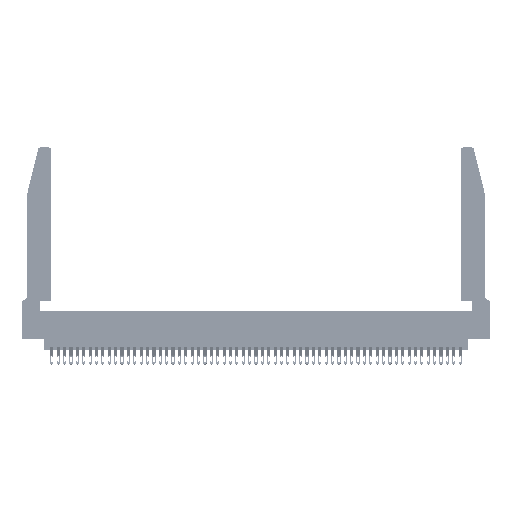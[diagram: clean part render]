
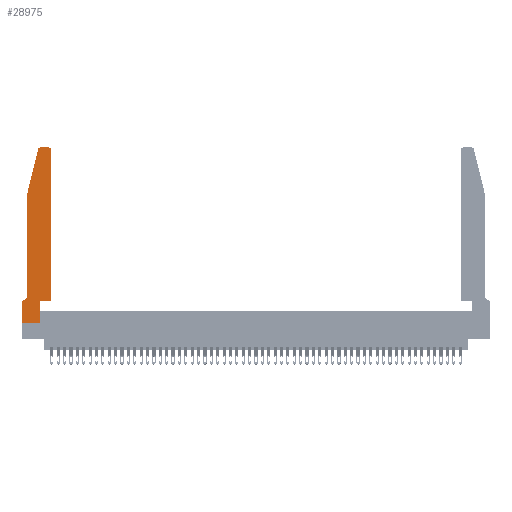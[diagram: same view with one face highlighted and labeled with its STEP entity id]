
A CAD part, top view. The second image highlights one B-rep face of the part: STEP entity #28975.
In plain terms, the highlighted planar face has unit normal (0, 0, 1).
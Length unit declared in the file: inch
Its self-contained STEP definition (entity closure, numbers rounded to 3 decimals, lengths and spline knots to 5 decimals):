
#190 = LINE ( 'NONE', #38748, #19589 ) ;
#1079 = CARTESIAN_POINT ( 'NONE',  ( 0.284, 2.72, 0.37 ) ) ;
#1463 = VERTEX_POINT ( 'NONE', #25729 ) ;
#1561 = CARTESIAN_POINT ( 'NONE',  ( 0., 0., 0.37 ) ) ;
#2939 = ORIENTED_EDGE ( 'NONE', *, *, #48172, .T. ) ;
#3310 = LINE ( 'NONE', #5385, #24082 ) ;
#4192 = ORIENTED_EDGE ( 'NONE', *, *, #30324, .T. ) ;
#4474 = CARTESIAN_POINT ( 'NONE',  ( 0.4205, 2.75, 0.37 ) ) ;
#5238 = DIRECTION ( 'NONE',  ( 1., 0., 0. ) ) ;
#5250 = EDGE_CURVE ( 'NONE', #14915, #1463, #14276, .T. ) ;
#5385 = CARTESIAN_POINT ( 'NONE',  ( 0.2865, 0.35, 0.37 ) ) ;
#6227 = CARTESIAN_POINT ( 'NONE',  ( 0.4505, 2.72, 0.37 ) ) ;
#6271 = CARTESIAN_POINT ( 'NONE',  ( 0.2865, 0., 0.37 ) ) ;
#6919 = VERTEX_POINT ( 'NONE', #47696 ) ;
#7175 = ORIENTED_EDGE ( 'NONE', *, *, #45312, .T. ) ;
#8162 = ORIENTED_EDGE ( 'NONE', *, *, #44693, .T. ) ;
#9348 = VECTOR ( 'NONE', #18435, 39.37008 ) ;
#9352 = CARTESIAN_POINT ( 'NONE',  ( 0.0755, 2., 0.37 ) ) ;
#9410 = VECTOR ( 'NONE', #16096, 39.37008 ) ;
#9532 = DIRECTION ( 'NONE',  ( 0., 1., 0. ) ) ;
#9596 = EDGE_CURVE ( 'NONE', #39973, #14915, #28061, .T. ) ;
#10187 = ORIENTED_EDGE ( 'NONE', *, *, #9596, .T. ) ;
#11005 = ORIENTED_EDGE ( 'NONE', *, *, #38860, .T. ) ;
#11355 = VECTOR ( 'NONE', #30906, 39.37008 ) ;
#11509 = CARTESIAN_POINT ( 'NONE',  ( 0.284, 2.75, 0.37 ) ) ;
#11606 = CARTESIAN_POINT ( 'NONE',  ( 0.4205, 2.72, 0.37 ) ) ;
#11788 = CARTESIAN_POINT ( 'NONE',  ( 0.0755, 2., 0.37 ) ) ;
#11971 = LINE ( 'NONE', #48693, #9410 ) ;
#12127 = DIRECTION ( 'NONE',  ( 0., 0., -1. ) ) ;
#12983 = EDGE_CURVE ( 'NONE', #33211, #14797, #50561, .T. ) ;
#13061 = VERTEX_POINT ( 'NONE', #1561 ) ;
#13498 = DIRECTION ( 'NONE',  ( -0.239, -0.971, 0. ) ) ;
#13992 = ORIENTED_EDGE ( 'NONE', *, *, #42454, .T. ) ;
#14218 = CARTESIAN_POINT ( 'NONE',  ( 0.0755, 0.35, 0.37 ) ) ;
#14276 = LINE ( 'NONE', #14218, #45751 ) ;
#14797 = VERTEX_POINT ( 'NONE', #11788 ) ;
#14915 = VERTEX_POINT ( 'NONE', #25037 ) ;
#15769 = DIRECTION ( 'NONE',  ( 1., 0., 0. ) ) ;
#16096 = DIRECTION ( 'NONE',  ( 0., -1., 0. ) ) ;
#17284 = AXIS2_PLACEMENT_3D ( 'NONE', #36824, #12127, #40929 ) ;
#18108 = VERTEX_POINT ( 'NONE', #27431 ) ;
#18251 = DIRECTION ( 'NONE',  ( -1., 0., 0. ) ) ;
#18422 = LINE ( 'NONE', #30812, #39003 ) ;
#18435 = DIRECTION ( 'NONE',  ( 0., 1., 0. ) ) ;
#18467 = CARTESIAN_POINT ( 'NONE',  ( 0., 0., 0.37 ) ) ;
#19589 = VECTOR ( 'NONE', #18251, 39.37008 ) ;
#19962 = EDGE_CURVE ( 'NONE', #13061, #19975, #33343, .T. ) ;
#19975 = VERTEX_POINT ( 'NONE', #6271 ) ;
#21295 = EDGE_CURVE ( 'NONE', #6919, #18108, #18422, .T. ) ;
#21751 = DIRECTION ( 'NONE',  ( 0., 0., 1. ) ) ;
#24082 = VECTOR ( 'NONE', #9532, 39.37008 ) ;
#25037 = CARTESIAN_POINT ( 'NONE',  ( 0.0055, 0.35, 0.37 ) ) ;
#25729 = CARTESIAN_POINT ( 'NONE',  ( 0., 0.35, 0.37 ) ) ;
#26739 = CARTESIAN_POINT ( 'NONE',  ( 0., 0., 0.37 ) ) ;
#27205 = ORIENTED_EDGE ( 'NONE', *, *, #19962, .T. ) ;
#27431 = CARTESIAN_POINT ( 'NONE',  ( 0.4505, 0.35, 0.37 ) ) ;
#27925 = VERTEX_POINT ( 'NONE', #6227 ) ;
#28061 = CIRCLE ( 'NONE', #17284, 0.07 ) ;
#28306 = EDGE_LOOP ( 'NONE', ( #8162, #4192, #49988, #11005, #10187, #47854, #2939, #27205, #7175, #41604, #43207, #13992 ) ) ;
#28964 = AXIS2_PLACEMENT_3D ( 'NONE', #46198, #21751, #50262 ) ;
#28975 = ADVANCED_FACE ( 'NONE', ( #33011 ), #29866, .T. ) ;
#29866 = PLANE ( 'NONE',  #28964 ) ;
#30067 = DIRECTION ( 'NONE',  ( 0., 0., 1. ) ) ;
#30324 = EDGE_CURVE ( 'NONE', #43581, #33211, #48127, .T. ) ;
#30812 = CARTESIAN_POINT ( 'NONE',  ( 0.4505, 0.35, 0.37 ) ) ;
#30906 = DIRECTION ( 'NONE',  ( 1., 0., 0. ) ) ;
#32078 = CARTESIAN_POINT ( 'NONE',  ( 0.0755, 0.42, 0.37 ) ) ;
#32955 = EDGE_CURVE ( 'NONE', #18108, #27925, #52905, .T. ) ;
#33011 = FACE_OUTER_BOUND ( 'NONE', #28306, .T. ) ;
#33211 = VERTEX_POINT ( 'NONE', #40491 ) ;
#33343 = LINE ( 'NONE', #26739, #11355 ) ;
#33853 = AXIS2_PLACEMENT_3D ( 'NONE', #1079, #30067, #5238 ) ;
#34854 = CARTESIAN_POINT ( 'NONE',  ( 0.4505, 0.35, 0.37 ) ) ;
#36532 = AXIS2_PLACEMENT_3D ( 'NONE', #11606, #40396, #15769 ) ;
#36824 = CARTESIAN_POINT ( 'NONE',  ( 0.0055, 0.42, 0.37 ) ) ;
#37909 = VECTOR ( 'NONE', #47308, 39.37008 ) ;
#38748 = CARTESIAN_POINT ( 'NONE',  ( 0.2605, 2.75, 0.37 ) ) ;
#38860 = EDGE_CURVE ( 'NONE', #14797, #39973, #11971, .T. ) ;
#38892 = DIRECTION ( 'NONE',  ( -1., 0., 0. ) ) ;
#38954 = DIRECTION ( 'NONE',  ( 1., 0., 0. ) ) ;
#39003 = VECTOR ( 'NONE', #38954, 39.37008 ) ;
#39748 = VECTOR ( 'NONE', #13498, 39.37008 ) ;
#39973 = VERTEX_POINT ( 'NONE', #32078 ) ;
#40396 = DIRECTION ( 'NONE',  ( 0., 0., 1. ) ) ;
#40491 = CARTESIAN_POINT ( 'NONE',  ( 0.25487, 2.72718, 0.37 ) ) ;
#40929 = DIRECTION ( 'NONE',  ( -1., 0., 0. ) ) ;
#41604 = ORIENTED_EDGE ( 'NONE', *, *, #21295, .T. ) ;
#42454 = EDGE_CURVE ( 'NONE', #27925, #45177, #43509, .T. ) ;
#43207 = ORIENTED_EDGE ( 'NONE', *, *, #32955, .T. ) ;
#43509 = CIRCLE ( 'NONE', #36532, 0.03 ) ;
#43581 = VERTEX_POINT ( 'NONE', #11509 ) ;
#44693 = EDGE_CURVE ( 'NONE', #45177, #43581, #190, .T. ) ;
#45177 = VERTEX_POINT ( 'NONE', #4474 ) ;
#45312 = EDGE_CURVE ( 'NONE', #19975, #6919, #3310, .T. ) ;
#45751 = VECTOR ( 'NONE', #38892, 39.37008 ) ;
#46198 = CARTESIAN_POINT ( 'NONE',  ( 0., 0.35, 0.37 ) ) ;
#47308 = DIRECTION ( 'NONE',  ( 0., -1., 0. ) ) ;
#47696 = CARTESIAN_POINT ( 'NONE',  ( 0.2865, 0.35, 0.37 ) ) ;
#47854 = ORIENTED_EDGE ( 'NONE', *, *, #5250, .T. ) ;
#48127 = CIRCLE ( 'NONE', #33853, 0.03 ) ;
#48172 = EDGE_CURVE ( 'NONE', #1463, #13061, #48660, .T. ) ;
#48660 = LINE ( 'NONE', #18467, #37909 ) ;
#48693 = CARTESIAN_POINT ( 'NONE',  ( 0.0755, 2., 0.37 ) ) ;
#49988 = ORIENTED_EDGE ( 'NONE', *, *, #12983, .T. ) ;
#50262 = DIRECTION ( 'NONE',  ( 1., 0., 0. ) ) ;
#50561 = LINE ( 'NONE', #9352, #39748 ) ;
#52905 = LINE ( 'NONE', #34854, #9348 ) ;
